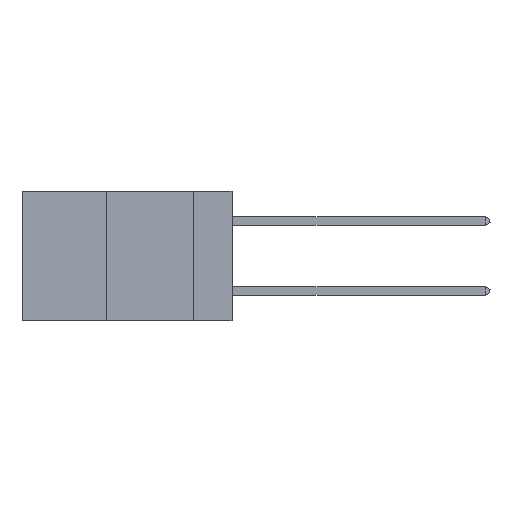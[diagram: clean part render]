
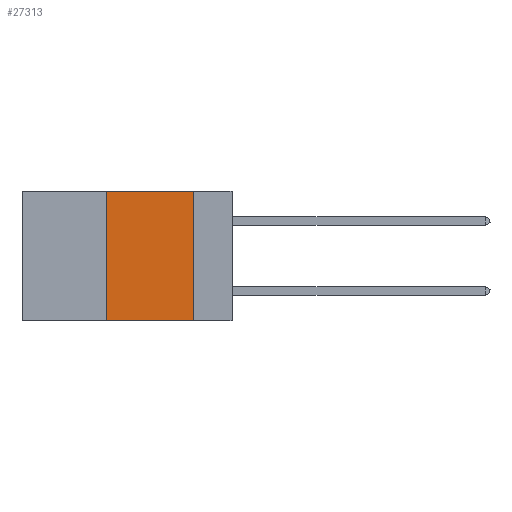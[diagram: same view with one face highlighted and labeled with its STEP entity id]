
A CAD part, left-side view. The second image highlights one B-rep face of the part: STEP entity #27313.
In plain terms, the highlighted planar face has unit normal (-1, 0, 0).
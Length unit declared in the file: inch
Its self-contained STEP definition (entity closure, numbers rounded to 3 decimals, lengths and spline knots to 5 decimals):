
#709 = VERTEX_POINT ( 'NONE', #22173 ) ;
#1032 = DIRECTION ( 'NONE',  ( 1., 0., 0. ) ) ;
#1964 = ORIENTED_EDGE ( 'NONE', *, *, #38630, .F. ) ;
#2819 = DIRECTION ( 'NONE',  ( 0., -1., 0. ) ) ;
#2967 = EDGE_CURVE ( 'NONE', #38922, #17266, #14790, .T. ) ;
#4565 = DIRECTION ( 'NONE',  ( 0., -1., 0. ) ) ;
#4590 = VERTEX_POINT ( 'NONE', #32724 ) ;
#6625 = DIRECTION ( 'NONE',  ( 0., 0., -1. ) ) ;
#6831 = AXIS2_PLACEMENT_3D ( 'NONE', #22175, #1032, #6625 ) ;
#11883 = CARTESIAN_POINT ( 'NONE',  ( 0., 0.6, 0. ) ) ;
#12033 = ORIENTED_EDGE ( 'NONE', *, *, #32132, .F. ) ;
#14458 = EDGE_LOOP ( 'NONE', ( #1964, #12033, #15499, #36376 ) ) ;
#14586 = VECTOR ( 'NONE', #2819, 39.37008 ) ;
#14790 = LINE ( 'NONE', #34984, #30540 ) ;
#15499 = ORIENTED_EDGE ( 'NONE', *, *, #33583, .F. ) ;
#16870 = VECTOR ( 'NONE', #33637, 39.37008 ) ;
#17266 = VERTEX_POINT ( 'NONE', #17716 ) ;
#17716 = CARTESIAN_POINT ( 'NONE',  ( 0., 0.11, -0.37 ) ) ;
#18811 = LINE ( 'NONE', #34153, #16870 ) ;
#20412 = LINE ( 'NONE', #11883, #14586 ) ;
#21979 = LINE ( 'NONE', #29087, #26724 ) ;
#22173 = CARTESIAN_POINT ( 'NONE',  ( 0., 0.36, 0. ) ) ;
#22175 = CARTESIAN_POINT ( 'NONE',  ( 0., 0.6, 0. ) ) ;
#23280 = DIRECTION ( 'NONE',  ( 0., 0., -1. ) ) ;
#26724 = VECTOR ( 'NONE', #23280, 39.37008 ) ;
#27313 = ADVANCED_FACE ( 'NONE', ( #33935 ), #31332, .F. ) ;
#29087 = CARTESIAN_POINT ( 'NONE',  ( 0., 0.11, 0. ) ) ;
#30540 = VECTOR ( 'NONE', #4565, 39.37008 ) ;
#31332 = PLANE ( 'NONE',  #6831 ) ;
#32132 = EDGE_CURVE ( 'NONE', #709, #4590, #20412, .T. ) ;
#32724 = CARTESIAN_POINT ( 'NONE',  ( 0., 0.11, 0. ) ) ;
#33583 = EDGE_CURVE ( 'NONE', #38922, #709, #18811, .T. ) ;
#33637 = DIRECTION ( 'NONE',  ( 0., 0., 1. ) ) ;
#33935 = FACE_OUTER_BOUND ( 'NONE', #14458, .T. ) ;
#34153 = CARTESIAN_POINT ( 'NONE',  ( 0., 0.36, 0. ) ) ;
#34984 = CARTESIAN_POINT ( 'NONE',  ( 0., 0.6, -0.37 ) ) ;
#36376 = ORIENTED_EDGE ( 'NONE', *, *, #2967, .T. ) ;
#36927 = CARTESIAN_POINT ( 'NONE',  ( 0., 0.36, -0.37 ) ) ;
#38630 = EDGE_CURVE ( 'NONE', #4590, #17266, #21979, .T. ) ;
#38922 = VERTEX_POINT ( 'NONE', #36927 ) ;
